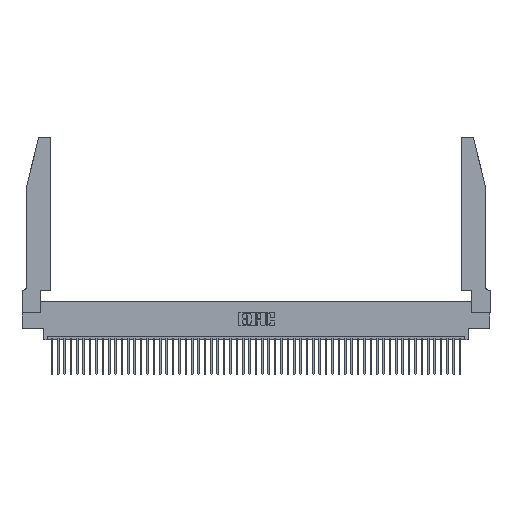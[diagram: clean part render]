
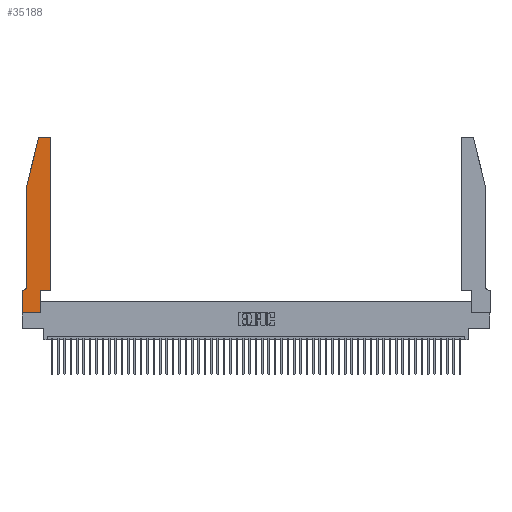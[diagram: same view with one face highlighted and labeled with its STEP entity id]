
A CAD part, top view. The second image highlights one B-rep face of the part: STEP entity #35188.
In plain terms, the highlighted planar face has unit normal (0, 0, 1).
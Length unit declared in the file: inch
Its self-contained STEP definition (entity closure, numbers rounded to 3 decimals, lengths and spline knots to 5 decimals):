
#412 = VERTEX_POINT ( 'NONE', #20236 ) ;
#669 = CARTESIAN_POINT ( 'NONE',  ( 0.0755, 2., 0.37 ) ) ;
#830 = LINE ( 'NONE', #29468, #20612 ) ;
#854 = EDGE_CURVE ( 'NONE', #50336, #46863, #51749, .T. ) ;
#1443 = ORIENTED_EDGE ( 'NONE', *, *, #50201, .T. ) ;
#1485 = CARTESIAN_POINT ( 'NONE',  ( 0.0755, 2., 0.37 ) ) ;
#1796 = DIRECTION ( 'NONE',  ( -1., 0., 0. ) ) ;
#2284 = VECTOR ( 'NONE', #29249, 39.37008 ) ;
#3599 = CARTESIAN_POINT ( 'NONE',  ( 0.2865, 0., 0.37 ) ) ;
#3814 = VERTEX_POINT ( 'NONE', #10973 ) ;
#3918 = VECTOR ( 'NONE', #9034, 39.37008 ) ;
#4133 = CARTESIAN_POINT ( 'NONE',  ( 0.0755, 0.42, 0.37 ) ) ;
#4385 = LINE ( 'NONE', #51457, #22873 ) ;
#4419 = DIRECTION ( 'NONE',  ( 0., 1., 0. ) ) ;
#4489 = DIRECTION ( 'NONE',  ( 1., 0., 0. ) ) ;
#4545 = VERTEX_POINT ( 'NONE', #13662 ) ;
#5221 = DIRECTION ( 'NONE',  ( 1., 0., 0. ) ) ;
#5523 = EDGE_CURVE ( 'NONE', #48755, #26769, #9302, .T. ) ;
#5576 = DIRECTION ( 'NONE',  ( 0., -1., 0. ) ) ;
#7307 = EDGE_CURVE ( 'NONE', #4545, #31475, #34089, .T. ) ;
#8267 = CARTESIAN_POINT ( 'NONE',  ( 0., 0.35, 0.37 ) ) ;
#9034 = DIRECTION ( 'NONE',  ( -0.239, -0.971, 0. ) ) ;
#9302 = LINE ( 'NONE', #32845, #2284 ) ;
#9569 = ORIENTED_EDGE ( 'NONE', *, *, #7307, .T. ) ;
#10123 = VECTOR ( 'NONE', #31984, 39.37008 ) ;
#10973 = CARTESIAN_POINT ( 'NONE',  ( 0.4505, 0.35, 0.37 ) ) ;
#12473 = AXIS2_PLACEMENT_3D ( 'NONE', #49970, #34126, #13560 ) ;
#12498 = VECTOR ( 'NONE', #5221, 39.37008 ) ;
#13034 = CARTESIAN_POINT ( 'NONE',  ( 0.284, 2.75, 0.37 ) ) ;
#13560 = DIRECTION ( 'NONE',  ( -1., 0., 0. ) ) ;
#13662 = CARTESIAN_POINT ( 'NONE',  ( 0.0755, 2., 0.37 ) ) ;
#13728 = CARTESIAN_POINT ( 'NONE',  ( 0.0755, 0.35, 0.37 ) ) ;
#15196 = EDGE_CURVE ( 'NONE', #19613, #412, #17656, .T. ) ;
#15547 = DIRECTION ( 'NONE',  ( 1., 0., 0. ) ) ;
#16895 = CARTESIAN_POINT ( 'NONE',  ( 0.2865, 0.35, 0.37 ) ) ;
#17335 = DIRECTION ( 'NONE',  ( 0., 0., 1. ) ) ;
#17340 = LINE ( 'NONE', #669, #3918 ) ;
#17342 = DIRECTION ( 'NONE',  ( -1., 0., 0. ) ) ;
#17656 = CIRCLE ( 'NONE', #23815, 0.03 ) ;
#18669 = CARTESIAN_POINT ( 'NONE',  ( 0.4205, 2.72, 0.37 ) ) ;
#18899 = EDGE_CURVE ( 'NONE', #412, #43817, #830, .T. ) ;
#19289 = ORIENTED_EDGE ( 'NONE', *, *, #45129, .T. ) ;
#19613 = VERTEX_POINT ( 'NONE', #38400 ) ;
#19898 = AXIS2_PLACEMENT_3D ( 'NONE', #28928, #17335, #4489 ) ;
#19944 = VERTEX_POINT ( 'NONE', #24723 ) ;
#20236 = CARTESIAN_POINT ( 'NONE',  ( 0.4205, 2.75, 0.37 ) ) ;
#20612 = VECTOR ( 'NONE', #17342, 39.37008 ) ;
#20968 = CARTESIAN_POINT ( 'NONE',  ( 0.0055, 0.35, 0.37 ) ) ;
#21267 = CARTESIAN_POINT ( 'NONE',  ( 0., 0.35, 0.37 ) ) ;
#22711 = VERTEX_POINT ( 'NONE', #20968 ) ;
#22873 = VECTOR ( 'NONE', #51808, 39.37008 ) ;
#23773 = VECTOR ( 'NONE', #5576, 39.37008 ) ;
#23815 = AXIS2_PLACEMENT_3D ( 'NONE', #18669, #50638, #50805 ) ;
#24723 = CARTESIAN_POINT ( 'NONE',  ( 0.25487, 2.72718, 0.37 ) ) ;
#25275 = ORIENTED_EDGE ( 'NONE', *, *, #48639, .T. ) ;
#25797 = AXIS2_PLACEMENT_3D ( 'NONE', #8267, #32174, #15547 ) ;
#26769 = VERTEX_POINT ( 'NONE', #33652 ) ;
#27604 = EDGE_CURVE ( 'NONE', #46863, #3814, #36125, .T. ) ;
#28928 = CARTESIAN_POINT ( 'NONE',  ( 0.284, 2.72, 0.37 ) ) ;
#29249 = DIRECTION ( 'NONE',  ( 0., -1., 0. ) ) ;
#29468 = CARTESIAN_POINT ( 'NONE',  ( 0.2605, 2.75, 0.37 ) ) ;
#29735 = ORIENTED_EDGE ( 'NONE', *, *, #27604, .T. ) ;
#31033 = ORIENTED_EDGE ( 'NONE', *, *, #854, .T. ) ;
#31475 = VERTEX_POINT ( 'NONE', #4133 ) ;
#31984 = DIRECTION ( 'NONE',  ( 0., 1., 0. ) ) ;
#32174 = DIRECTION ( 'NONE',  ( 0., 0., 1. ) ) ;
#32845 = CARTESIAN_POINT ( 'NONE',  ( 0., 0., 0.37 ) ) ;
#33652 = CARTESIAN_POINT ( 'NONE',  ( 0., 0., 0.37 ) ) ;
#33718 = ORIENTED_EDGE ( 'NONE', *, *, #34920, .T. ) ;
#34089 = LINE ( 'NONE', #1485, #23773 ) ;
#34126 = DIRECTION ( 'NONE',  ( 0., 0., -1. ) ) ;
#34920 = EDGE_CURVE ( 'NONE', #22711, #48755, #43507, .T. ) ;
#35188 = ADVANCED_FACE ( 'NONE', ( #51103 ), #40789, .T. ) ;
#35318 = ORIENTED_EDGE ( 'NONE', *, *, #15196, .T. ) ;
#36125 = LINE ( 'NONE', #50155, #12498 ) ;
#36910 = CARTESIAN_POINT ( 'NONE',  ( 0.2865, 0.35, 0.37 ) ) ;
#36975 = ORIENTED_EDGE ( 'NONE', *, *, #18899, .T. ) ;
#38400 = CARTESIAN_POINT ( 'NONE',  ( 0.4505, 2.72, 0.37 ) ) ;
#39546 = EDGE_LOOP ( 'NONE', ( #36975, #25275, #19289, #9569, #44724, #33718, #43161, #1443, #31033, #29735, #43695, #35318 ) ) ;
#40345 = EDGE_CURVE ( 'NONE', #31475, #22711, #49009, .T. ) ;
#40789 = PLANE ( 'NONE',  #25797 ) ;
#42270 = VECTOR ( 'NONE', #4419, 39.37008 ) ;
#43161 = ORIENTED_EDGE ( 'NONE', *, *, #5523, .T. ) ;
#43507 = LINE ( 'NONE', #13728, #50465 ) ;
#43695 = ORIENTED_EDGE ( 'NONE', *, *, #50435, .T. ) ;
#43817 = VERTEX_POINT ( 'NONE', #13034 ) ;
#44182 = CARTESIAN_POINT ( 'NONE',  ( 0.4505, 0.35, 0.37 ) ) ;
#44724 = ORIENTED_EDGE ( 'NONE', *, *, #40345, .T. ) ;
#45129 = EDGE_CURVE ( 'NONE', #19944, #4545, #17340, .T. ) ;
#46471 = CIRCLE ( 'NONE', #19898, 0.03 ) ;
#46863 = VERTEX_POINT ( 'NONE', #36910 ) ;
#48417 = LINE ( 'NONE', #44182, #10123 ) ;
#48639 = EDGE_CURVE ( 'NONE', #43817, #19944, #46471, .T. ) ;
#48755 = VERTEX_POINT ( 'NONE', #21267 ) ;
#49009 = CIRCLE ( 'NONE', #12473, 0.07 ) ;
#49970 = CARTESIAN_POINT ( 'NONE',  ( 0.0055, 0.42, 0.37 ) ) ;
#50155 = CARTESIAN_POINT ( 'NONE',  ( 0.4505, 0.35, 0.37 ) ) ;
#50201 = EDGE_CURVE ( 'NONE', #26769, #50336, #4385, .T. ) ;
#50336 = VERTEX_POINT ( 'NONE', #3599 ) ;
#50435 = EDGE_CURVE ( 'NONE', #3814, #19613, #48417, .T. ) ;
#50465 = VECTOR ( 'NONE', #1796, 39.37008 ) ;
#50638 = DIRECTION ( 'NONE',  ( 0., 0., 1. ) ) ;
#50805 = DIRECTION ( 'NONE',  ( 1., 0., 0. ) ) ;
#51103 = FACE_OUTER_BOUND ( 'NONE', #39546, .T. ) ;
#51457 = CARTESIAN_POINT ( 'NONE',  ( 0., 0., 0.37 ) ) ;
#51749 = LINE ( 'NONE', #16895, #42270 ) ;
#51808 = DIRECTION ( 'NONE',  ( 1., 0., 0. ) ) ;
